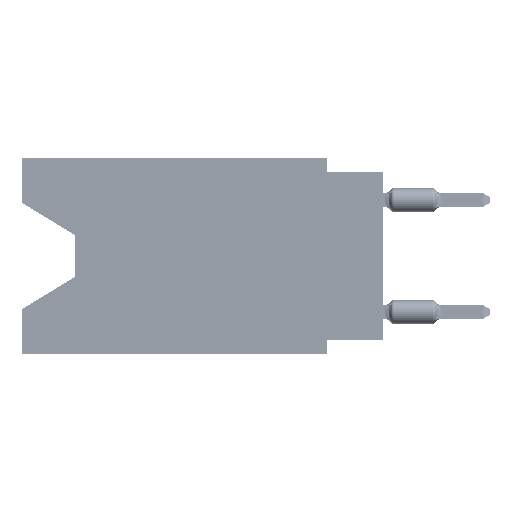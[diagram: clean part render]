
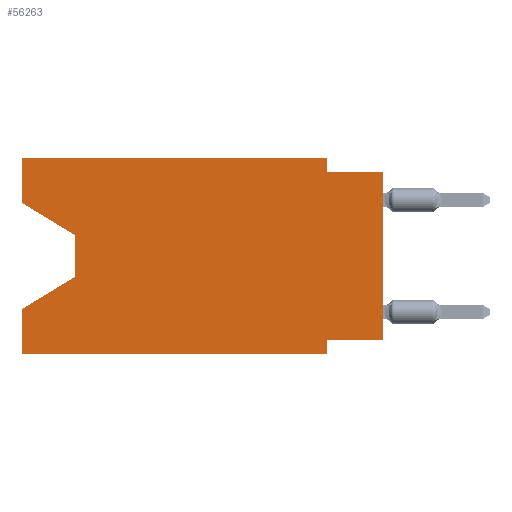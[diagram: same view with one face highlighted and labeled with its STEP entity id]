
A CAD part, left-side view. The second image highlights one B-rep face of the part: STEP entity #56263.
In plain terms, the highlighted planar face has unit normal (-1, 0, 0).
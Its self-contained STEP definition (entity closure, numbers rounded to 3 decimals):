
#443 = CARTESIAN_POINT ( 'NONE',  ( 0., 2.54, -8.89 ) ) ;
#1016 = ORIENTED_EDGE ( 'NONE', *, *, #12600, .F. ) ;
#2565 = ORIENTED_EDGE ( 'NONE', *, *, #36635, .T. ) ;
#2966 = EDGE_CURVE ( 'NONE', #63494, #65078, #25461, .T. ) ;
#4245 = CARTESIAN_POINT ( 'NONE',  ( 0., 2.54, 0. ) ) ;
#4346 = CARTESIAN_POINT ( 'NONE',  ( 0., 16.383, -2.038 ) ) ;
#4465 = DIRECTION ( 'NONE',  ( 0., -1., 0. ) ) ;
#4755 = VECTOR ( 'NONE', #33260, 1000. ) ;
#5250 = EDGE_CURVE ( 'NONE', #10993, #63494, #58230, .T. ) ;
#5744 = VERTEX_POINT ( 'NONE', #36905 ) ;
#5791 = CARTESIAN_POINT ( 'NONE',  ( 0., 16.383, -6.852 ) ) ;
#7074 = AXIS2_PLACEMENT_3D ( 'NONE', #54995, #21904, #33051 ) ;
#7410 = PLANE ( 'NONE',  #7074 ) ;
#8643 = EDGE_CURVE ( 'NONE', #5744, #14140, #62868, .T. ) ;
#9614 = LINE ( 'NONE', #4245, #17934 ) ;
#10195 = CARTESIAN_POINT ( 'NONE',  ( 0., 16.383, 0. ) ) ;
#10993 = VERTEX_POINT ( 'NONE', #4346 ) ;
#11344 = CARTESIAN_POINT ( 'NONE',  ( 0., 16.383, 0. ) ) ;
#12419 = VECTOR ( 'NONE', #41519, 1000. ) ;
#12600 = EDGE_CURVE ( 'NONE', #13275, #28866, #46570, .T. ) ;
#12767 = CARTESIAN_POINT ( 'NONE',  ( 0., 16.383, 0. ) ) ;
#13187 = LINE ( 'NONE', #45545, #51481 ) ;
#13275 = VERTEX_POINT ( 'NONE', #12767 ) ;
#13449 = EDGE_CURVE ( 'NONE', #5744, #45875, #27701, .T. ) ;
#13508 = CARTESIAN_POINT ( 'NONE',  ( 0., 16.383, 0. ) ) ;
#13581 = CARTESIAN_POINT ( 'NONE',  ( 0., 13.97, -5.385 ) ) ;
#13638 = CARTESIAN_POINT ( 'NONE',  ( 0., 13.97, -3.505 ) ) ;
#14140 = VERTEX_POINT ( 'NONE', #30846 ) ;
#14168 = LINE ( 'NONE', #31777, #43512 ) ;
#14269 = EDGE_CURVE ( 'NONE', #28866, #24029, #9614, .T. ) ;
#15819 = CARTESIAN_POINT ( 'NONE',  ( 0., 2.54, -0.635 ) ) ;
#15946 = ORIENTED_EDGE ( 'NONE', *, *, #2966, .T. ) ;
#17934 = VECTOR ( 'NONE', #26156, 1000. ) ;
#18225 = DIRECTION ( 'NONE',  ( 0., -1., 0. ) ) ;
#18602 = VERTEX_POINT ( 'NONE', #5791 ) ;
#18802 = VECTOR ( 'NONE', #20118, 1000. ) ;
#18861 = CARTESIAN_POINT ( 'NONE',  ( 0., 0., -0.635 ) ) ;
#19604 = CARTESIAN_POINT ( 'NONE',  ( 0., 0., 0. ) ) ;
#20118 = DIRECTION ( 'NONE',  ( 0., -0.855, -0.519 ) ) ;
#21904 = DIRECTION ( 'NONE',  ( 1., 0., 0. ) ) ;
#23464 = CARTESIAN_POINT ( 'NONE',  ( 0., 2.54, -8.89 ) ) ;
#24029 = VERTEX_POINT ( 'NONE', #15819 ) ;
#25461 = LINE ( 'NONE', #13638, #48566 ) ;
#26156 = DIRECTION ( 'NONE',  ( 0., 0., -1. ) ) ;
#26910 = CARTESIAN_POINT ( 'NONE',  ( 0., 2.54, 0. ) ) ;
#27040 = ORIENTED_EDGE ( 'NONE', *, *, #60940, .F. ) ;
#27514 = LINE ( 'NONE', #11344, #4755 ) ;
#27701 = LINE ( 'NONE', #19604, #12419 ) ;
#28031 = CARTESIAN_POINT ( 'NONE',  ( 0., 16.383, -8.89 ) ) ;
#28852 = LINE ( 'NONE', #23464, #36221 ) ;
#28866 = VERTEX_POINT ( 'NONE', #26910 ) ;
#30846 = CARTESIAN_POINT ( 'NONE',  ( 0., 2.54, -8.255 ) ) ;
#31777 = CARTESIAN_POINT ( 'NONE',  ( 0., 16.383, -8.89 ) ) ;
#32970 = EDGE_CURVE ( 'NONE', #43421, #18602, #27514, .T. ) ;
#33051 = DIRECTION ( 'NONE',  ( 0., 0., -1. ) ) ;
#33089 = VECTOR ( 'NONE', #57460, 1000. ) ;
#33260 = DIRECTION ( 'NONE',  ( 0., 0., 1. ) ) ;
#35525 = CARTESIAN_POINT ( 'NONE',  ( 0., 0., -8.255 ) ) ;
#36221 = VECTOR ( 'NONE', #45400, 1000. ) ;
#36635 = EDGE_CURVE ( 'NONE', #65078, #18602, #62826, .T. ) ;
#36905 = CARTESIAN_POINT ( 'NONE',  ( 0., 0., -8.255 ) ) ;
#40487 = ORIENTED_EDGE ( 'NONE', *, *, #69838, .F. ) ;
#41008 = ORIENTED_EDGE ( 'NONE', *, *, #14269, .F. ) ;
#41519 = DIRECTION ( 'NONE',  ( 0., 0., 1. ) ) ;
#41524 = VECTOR ( 'NONE', #42544, 1000. ) ;
#41532 = EDGE_CURVE ( 'NONE', #10993, #13275, #53710, .T. ) ;
#42434 = EDGE_LOOP ( 'NONE', ( #60915, #15946, #2565, #55697, #44311, #27040, #67718, #56173, #40487, #41008, #1016, #52456 ) ) ;
#42544 = DIRECTION ( 'NONE',  ( 0., 0., 1. ) ) ;
#42810 = VECTOR ( 'NONE', #67773, 1000. ) ;
#43421 = VERTEX_POINT ( 'NONE', #28031 ) ;
#43512 = VECTOR ( 'NONE', #4465, 1000. ) ;
#44311 = ORIENTED_EDGE ( 'NONE', *, *, #70373, .T. ) ;
#45400 = DIRECTION ( 'NONE',  ( 0., 0., -1. ) ) ;
#45545 = CARTESIAN_POINT ( 'NONE',  ( 0., 0., -0.635 ) ) ;
#45875 = VERTEX_POINT ( 'NONE', #18861 ) ;
#46570 = LINE ( 'NONE', #13508, #42810 ) ;
#47410 = DIRECTION ( 'NONE',  ( 0., 0., -1. ) ) ;
#48566 = VECTOR ( 'NONE', #47410, 1000. ) ;
#49580 = FACE_OUTER_BOUND ( 'NONE', #42434, .T. ) ;
#50600 = CARTESIAN_POINT ( 'NONE',  ( 0., 13.97, -5.385 ) ) ;
#51481 = VECTOR ( 'NONE', #18225, 1000. ) ;
#52456 = ORIENTED_EDGE ( 'NONE', *, *, #41532, .F. ) ;
#53710 = LINE ( 'NONE', #10195, #41524 ) ;
#54995 = CARTESIAN_POINT ( 'NONE',  ( 0., 16.383, 0. ) ) ;
#55697 = ORIENTED_EDGE ( 'NONE', *, *, #32970, .F. ) ;
#56173 = ORIENTED_EDGE ( 'NONE', *, *, #13449, .T. ) ;
#56263 = ADVANCED_FACE ( 'NONE', ( #49580 ), #7410, .F. ) ;
#57460 = DIRECTION ( 'NONE',  ( 0., 1., 0. ) ) ;
#58230 = LINE ( 'NONE', #68672, #18802 ) ;
#60622 = VECTOR ( 'NONE', #62458, 1000. ) ;
#60915 = ORIENTED_EDGE ( 'NONE', *, *, #5250, .T. ) ;
#60940 = EDGE_CURVE ( 'NONE', #14140, #68804, #28852, .T. ) ;
#62458 = DIRECTION ( 'NONE',  ( 0., 0.855, -0.519 ) ) ;
#62826 = LINE ( 'NONE', #13581, #60622 ) ;
#62868 = LINE ( 'NONE', #35525, #33089 ) ;
#63126 = CARTESIAN_POINT ( 'NONE',  ( 0., 13.97, -3.505 ) ) ;
#63494 = VERTEX_POINT ( 'NONE', #63126 ) ;
#65078 = VERTEX_POINT ( 'NONE', #50600 ) ;
#67718 = ORIENTED_EDGE ( 'NONE', *, *, #8643, .F. ) ;
#67773 = DIRECTION ( 'NONE',  ( 0., -1., 0. ) ) ;
#68672 = CARTESIAN_POINT ( 'NONE',  ( 0., 16.383, -2.038 ) ) ;
#68804 = VERTEX_POINT ( 'NONE', #443 ) ;
#69838 = EDGE_CURVE ( 'NONE', #24029, #45875, #13187, .T. ) ;
#70373 = EDGE_CURVE ( 'NONE', #43421, #68804, #14168, .T. ) ;
